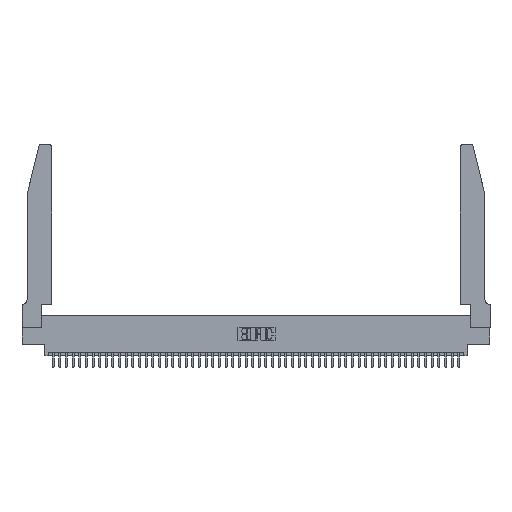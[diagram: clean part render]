
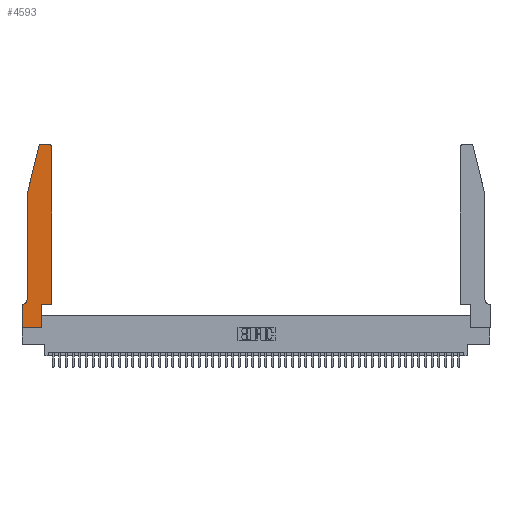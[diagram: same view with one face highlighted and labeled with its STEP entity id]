
A CAD part, top view. The second image highlights one B-rep face of the part: STEP entity #4593.
In plain terms, the highlighted planar face has unit normal (0, 0, 1).
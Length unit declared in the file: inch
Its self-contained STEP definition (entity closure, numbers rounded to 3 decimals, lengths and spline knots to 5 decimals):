
#359 = DIRECTION ( 'NONE',  ( 0., 0., 1. ) ) ;
#474 = CARTESIAN_POINT ( 'NONE',  ( 0.0755, 2., 0.37 ) ) ;
#900 = ORIENTED_EDGE ( 'NONE', *, *, #25739, .T. ) ;
#1058 = VERTEX_POINT ( 'NONE', #35119 ) ;
#1065 = CARTESIAN_POINT ( 'NONE',  ( 0., 0., 0.37 ) ) ;
#1213 = EDGE_CURVE ( 'NONE', #38094, #19848, #50638, .T. ) ;
#1365 = EDGE_LOOP ( 'NONE', ( #38419, #900, #31004, #45801, #30467, #5871, #33660, #38546, #9038, #49825, #50172, #2005 ) ) ;
#2005 = ORIENTED_EDGE ( 'NONE', *, *, #47139, .T. ) ;
#2178 = VECTOR ( 'NONE', #40511, 39.37008 ) ;
#2418 = EDGE_CURVE ( 'NONE', #48918, #3734, #24049, .T. ) ;
#2567 = CARTESIAN_POINT ( 'NONE',  ( 0.4205, 2.72, 0.37 ) ) ;
#3038 = CARTESIAN_POINT ( 'NONE',  ( 0.4505, 0.35, 0.37 ) ) ;
#3734 = VERTEX_POINT ( 'NONE', #27101 ) ;
#3774 = CARTESIAN_POINT ( 'NONE',  ( 0.4505, 2.72, 0.37 ) ) ;
#3917 = CARTESIAN_POINT ( 'NONE',  ( 0.0755, 0.42, 0.37 ) ) ;
#4593 = ADVANCED_FACE ( 'NONE', ( #30351 ), #19976, .T. ) ;
#5871 = ORIENTED_EDGE ( 'NONE', *, *, #16060, .T. ) ;
#6508 = DIRECTION ( 'NONE',  ( 1., 0., 0. ) ) ;
#7059 = CARTESIAN_POINT ( 'NONE',  ( 0.2605, 2.75, 0.37 ) ) ;
#7181 = AXIS2_PLACEMENT_3D ( 'NONE', #2567, #30088, #6508 ) ;
#7185 = LINE ( 'NONE', #29677, #16478 ) ;
#7594 = CARTESIAN_POINT ( 'NONE',  ( 0.284, 2.72, 0.37 ) ) ;
#9038 = ORIENTED_EDGE ( 'NONE', *, *, #15415, .T. ) ;
#9547 = EDGE_CURVE ( 'NONE', #19848, #31017, #14529, .T. ) ;
#9797 = EDGE_CURVE ( 'NONE', #1058, #34869, #12658, .T. ) ;
#10595 = VERTEX_POINT ( 'NONE', #26430 ) ;
#11263 = VECTOR ( 'NONE', #16002, 39.37008 ) ;
#11556 = DIRECTION ( 'NONE',  ( 1., 0., 0. ) ) ;
#12032 = VERTEX_POINT ( 'NONE', #3774 ) ;
#12441 = CIRCLE ( 'NONE', #33612, 0.03 ) ;
#12658 = LINE ( 'NONE', #1065, #2178 ) ;
#14027 = DIRECTION ( 'NONE',  ( 1., 0., 0. ) ) ;
#14529 = CIRCLE ( 'NONE', #31157, 0.07 ) ;
#15063 = CARTESIAN_POINT ( 'NONE',  ( 0.0055, 0.42, 0.37 ) ) ;
#15415 = EDGE_CURVE ( 'NONE', #34869, #33010, #7185, .T. ) ;
#15823 = VERTEX_POINT ( 'NONE', #19635 ) ;
#16002 = DIRECTION ( 'NONE',  ( 0., -1., 0. ) ) ;
#16060 = EDGE_CURVE ( 'NONE', #31017, #10595, #28671, .T. ) ;
#16478 = VECTOR ( 'NONE', #33682, 39.37008 ) ;
#16668 = CARTESIAN_POINT ( 'NONE',  ( 0.4205, 2.75, 0.37 ) ) ;
#17828 = CARTESIAN_POINT ( 'NONE',  ( 0.4505, 0.35, 0.37 ) ) ;
#18975 = DIRECTION ( 'NONE',  ( -1., 0., 0. ) ) ;
#19635 = CARTESIAN_POINT ( 'NONE',  ( 0.4505, 0.35, 0.37 ) ) ;
#19848 = VERTEX_POINT ( 'NONE', #3917 ) ;
#19976 = PLANE ( 'NONE',  #39656 ) ;
#21135 = VECTOR ( 'NONE', #23182, 39.37008 ) ;
#23182 = DIRECTION ( 'NONE',  ( -0.239, -0.971, 0. ) ) ;
#24049 = LINE ( 'NONE', #7059, #34545 ) ;
#25739 = EDGE_CURVE ( 'NONE', #3734, #28005, #12441, .T. ) ;
#26430 = CARTESIAN_POINT ( 'NONE',  ( 0., 0.35, 0.37 ) ) ;
#26682 = DIRECTION ( 'NONE',  ( -1., 0., 0. ) ) ;
#27101 = CARTESIAN_POINT ( 'NONE',  ( 0.284, 2.75, 0.37 ) ) ;
#27864 = CARTESIAN_POINT ( 'NONE',  ( 0., 0., 0.37 ) ) ;
#27900 = DIRECTION ( 'NONE',  ( 1., 0., 0. ) ) ;
#28005 = VERTEX_POINT ( 'NONE', #50113 ) ;
#28168 = CARTESIAN_POINT ( 'NONE',  ( 0.0055, 0.35, 0.37 ) ) ;
#28669 = CARTESIAN_POINT ( 'NONE',  ( 0.2865, 0.35, 0.37 ) ) ;
#28671 = LINE ( 'NONE', #28907, #48355 ) ;
#28907 = CARTESIAN_POINT ( 'NONE',  ( 0.0755, 0.35, 0.37 ) ) ;
#28997 = EDGE_CURVE ( 'NONE', #10595, #1058, #42984, .T. ) ;
#29677 = CARTESIAN_POINT ( 'NONE',  ( 0.2865, 0.35, 0.37 ) ) ;
#30088 = DIRECTION ( 'NONE',  ( 0., 0., 1. ) ) ;
#30304 = VECTOR ( 'NONE', #46382, 39.37008 ) ;
#30351 = FACE_OUTER_BOUND ( 'NONE', #1365, .T. ) ;
#30467 = ORIENTED_EDGE ( 'NONE', *, *, #9547, .T. ) ;
#30821 = VECTOR ( 'NONE', #14027, 39.37008 ) ;
#31004 = ORIENTED_EDGE ( 'NONE', *, *, #42855, .T. ) ;
#31017 = VERTEX_POINT ( 'NONE', #28168 ) ;
#31157 = AXIS2_PLACEMENT_3D ( 'NONE', #15063, #42591, #18975 ) ;
#32869 = LINE ( 'NONE', #34942, #21135 ) ;
#33010 = VERTEX_POINT ( 'NONE', #28669 ) ;
#33612 = AXIS2_PLACEMENT_3D ( 'NONE', #7594, #35163, #11556 ) ;
#33660 = ORIENTED_EDGE ( 'NONE', *, *, #28997, .T. ) ;
#33682 = DIRECTION ( 'NONE',  ( 0., 1., 0. ) ) ;
#34255 = CIRCLE ( 'NONE', #7181, 0.03 ) ;
#34545 = VECTOR ( 'NONE', #26682, 39.37008 ) ;
#34869 = VERTEX_POINT ( 'NONE', #46841 ) ;
#34942 = CARTESIAN_POINT ( 'NONE',  ( 0.0755, 2., 0.37 ) ) ;
#35119 = CARTESIAN_POINT ( 'NONE',  ( 0., 0., 0.37 ) ) ;
#35163 = DIRECTION ( 'NONE',  ( 0., 0., 1. ) ) ;
#36154 = DIRECTION ( 'NONE',  ( 0., -1., 0. ) ) ;
#36882 = DIRECTION ( 'NONE',  ( -1., 0., 0. ) ) ;
#38094 = VERTEX_POINT ( 'NONE', #38725 ) ;
#38419 = ORIENTED_EDGE ( 'NONE', *, *, #2418, .T. ) ;
#38546 = ORIENTED_EDGE ( 'NONE', *, *, #9797, .T. ) ;
#38725 = CARTESIAN_POINT ( 'NONE',  ( 0.0755, 2., 0.37 ) ) ;
#39656 = AXIS2_PLACEMENT_3D ( 'NONE', #47497, #359, #27900 ) ;
#40511 = DIRECTION ( 'NONE',  ( 1., 0., 0. ) ) ;
#40693 = EDGE_CURVE ( 'NONE', #33010, #15823, #41331, .T. ) ;
#40824 = LINE ( 'NONE', #3038, #30304 ) ;
#41331 = LINE ( 'NONE', #17828, #30821 ) ;
#42591 = DIRECTION ( 'NONE',  ( 0., 0., -1. ) ) ;
#42855 = EDGE_CURVE ( 'NONE', #28005, #38094, #32869, .T. ) ;
#42984 = LINE ( 'NONE', #27864, #50943 ) ;
#43331 = EDGE_CURVE ( 'NONE', #15823, #12032, #40824, .T. ) ;
#45801 = ORIENTED_EDGE ( 'NONE', *, *, #1213, .T. ) ;
#46382 = DIRECTION ( 'NONE',  ( 0., 1., 0. ) ) ;
#46841 = CARTESIAN_POINT ( 'NONE',  ( 0.2865, 0., 0.37 ) ) ;
#47139 = EDGE_CURVE ( 'NONE', #12032, #48918, #34255, .T. ) ;
#47497 = CARTESIAN_POINT ( 'NONE',  ( 0., 0.35, 0.37 ) ) ;
#48355 = VECTOR ( 'NONE', #36882, 39.37008 ) ;
#48918 = VERTEX_POINT ( 'NONE', #16668 ) ;
#49825 = ORIENTED_EDGE ( 'NONE', *, *, #40693, .T. ) ;
#50113 = CARTESIAN_POINT ( 'NONE',  ( 0.25487, 2.72718, 0.37 ) ) ;
#50172 = ORIENTED_EDGE ( 'NONE', *, *, #43331, .T. ) ;
#50638 = LINE ( 'NONE', #474, #11263 ) ;
#50943 = VECTOR ( 'NONE', #36154, 39.37008 ) ;
